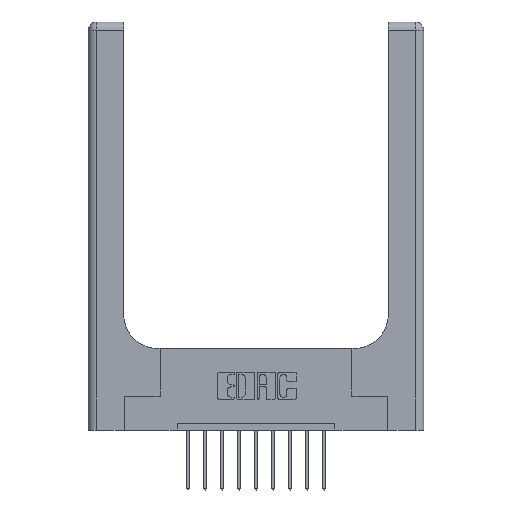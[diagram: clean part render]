
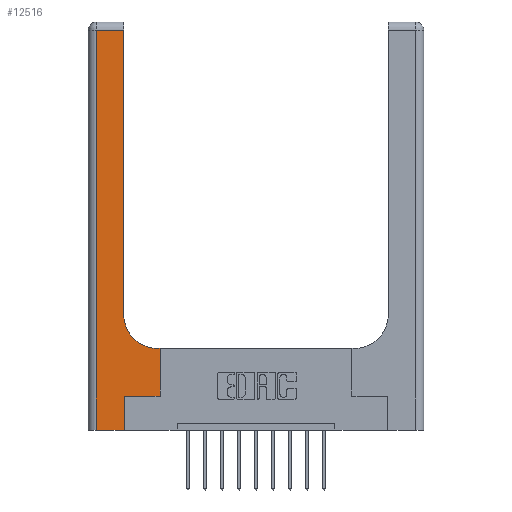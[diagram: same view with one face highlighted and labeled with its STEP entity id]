
A CAD part, top view. The second image highlights one B-rep face of the part: STEP entity #12516.
In plain terms, the highlighted planar face has unit normal (0, 0, 1).
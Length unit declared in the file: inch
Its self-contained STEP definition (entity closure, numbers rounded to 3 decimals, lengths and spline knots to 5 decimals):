
#198 = LINE ( 'NONE', #5008, #10710 ) ;
#617 = DIRECTION ( 'NONE',  ( 0., 0., -1. ) ) ;
#847 = VERTEX_POINT ( 'NONE', #10079 ) ;
#943 = EDGE_CURVE ( 'NONE', #5812, #9775, #3276, .T. ) ;
#958 = EDGE_LOOP ( 'NONE', ( #9670, #5380, #9196, #5825, #5721, #4698, #2646, #11241, #13419 ) ) ;
#1490 = CARTESIAN_POINT ( 'NONE',  ( 0.26, 2.94, 0.37 ) ) ;
#1755 = VERTEX_POINT ( 'NONE', #4124 ) ;
#2217 = LINE ( 'NONE', #7058, #12520 ) ;
#2228 = CARTESIAN_POINT ( 'NONE',  ( 0.265, 0., 0.37 ) ) ;
#2293 = VERTEX_POINT ( 'NONE', #7023 ) ;
#2319 = VECTOR ( 'NONE', #10686, 39.37008 ) ;
#2527 = EDGE_CURVE ( 'NONE', #1755, #2293, #14695, .T. ) ;
#2646 = ORIENTED_EDGE ( 'NONE', *, *, #2527, .T. ) ;
#3151 = LINE ( 'NONE', #15145, #7946 ) ;
#3276 = LINE ( 'NONE', #9407, #2319 ) ;
#3753 = VERTEX_POINT ( 'NONE', #9052 ) ;
#3847 = FACE_OUTER_BOUND ( 'NONE', #958, .T. ) ;
#4062 = VERTEX_POINT ( 'NONE', #7925 ) ;
#4124 = CARTESIAN_POINT ( 'NONE',  ( 0.528, 0.25, 0.37 ) ) ;
#4272 = DIRECTION ( 'NONE',  ( -1., 0., 0. ) ) ;
#4309 = DIRECTION ( 'NONE',  ( -1., 0., 0. ) ) ;
#4390 = CARTESIAN_POINT ( 'NONE',  ( 0.26, 0.6, 0.37 ) ) ;
#4558 = VERTEX_POINT ( 'NONE', #15347 ) ;
#4698 = ORIENTED_EDGE ( 'NONE', *, *, #9239, .T. ) ;
#5008 = CARTESIAN_POINT ( 'NONE',  ( 0., 0., 0.37 ) ) ;
#5085 = DIRECTION ( 'NONE',  ( 0., 1., 0. ) ) ;
#5380 = ORIENTED_EDGE ( 'NONE', *, *, #9116, .T. ) ;
#5564 = LINE ( 'NONE', #2228, #12491 ) ;
#5721 = ORIENTED_EDGE ( 'NONE', *, *, #13725, .T. ) ;
#5812 = VERTEX_POINT ( 'NONE', #6152 ) ;
#5825 = ORIENTED_EDGE ( 'NONE', *, *, #8790, .T. ) ;
#5881 = DIRECTION ( 'NONE',  ( 0., 1., 0. ) ) ;
#6116 = EDGE_CURVE ( 'NONE', #847, #4062, #7657, .T. ) ;
#6152 = CARTESIAN_POINT ( 'NONE',  ( 0.26, 0.85, 0.37 ) ) ;
#6202 = CARTESIAN_POINT ( 'NONE',  ( 0.528, 0.25, 0.37 ) ) ;
#6392 = DIRECTION ( 'NONE',  ( 1., 0., 0. ) ) ;
#6545 = AXIS2_PLACEMENT_3D ( 'NONE', #9834, #13670, #8715 ) ;
#7001 = AXIS2_PLACEMENT_3D ( 'NONE', #10214, #617, #6392 ) ;
#7023 = CARTESIAN_POINT ( 'NONE',  ( 0.528, 0.6, 0.37 ) ) ;
#7058 = CARTESIAN_POINT ( 'NONE',  ( 0.265, 0.25, 0.37 ) ) ;
#7136 = DIRECTION ( 'NONE',  ( 1., 0., 0. ) ) ;
#7339 = LINE ( 'NONE', #4390, #8923 ) ;
#7657 = LINE ( 'NONE', #15008, #14928 ) ;
#7925 = CARTESIAN_POINT ( 'NONE',  ( 0.06, 0., 0.37 ) ) ;
#7946 = VECTOR ( 'NONE', #4272, 39.37008 ) ;
#8444 = VECTOR ( 'NONE', #5085, 39.37008 ) ;
#8715 = DIRECTION ( 'NONE',  ( -1., 0., 0. ) ) ;
#8790 = EDGE_CURVE ( 'NONE', #4062, #3753, #198, .T. ) ;
#8923 = VECTOR ( 'NONE', #4309, 39.37008 ) ;
#9052 = CARTESIAN_POINT ( 'NONE',  ( 0.265, 0., 0.37 ) ) ;
#9116 = EDGE_CURVE ( 'NONE', #9775, #847, #3151, .T. ) ;
#9196 = ORIENTED_EDGE ( 'NONE', *, *, #6116, .T. ) ;
#9239 = EDGE_CURVE ( 'NONE', #12448, #1755, #2217, .T. ) ;
#9407 = CARTESIAN_POINT ( 'NONE',  ( 0.26, 3., 0.37 ) ) ;
#9670 = ORIENTED_EDGE ( 'NONE', *, *, #943, .T. ) ;
#9775 = VERTEX_POINT ( 'NONE', #1490 ) ;
#9834 = CARTESIAN_POINT ( 'NONE',  ( 0., 3., 0.37 ) ) ;
#10079 = CARTESIAN_POINT ( 'NONE',  ( 0.06, 2.94, 0.37 ) ) ;
#10118 = DIRECTION ( 'NONE',  ( 0., -1., 0. ) ) ;
#10214 = CARTESIAN_POINT ( 'NONE',  ( 0.51, 0.85, 0.37 ) ) ;
#10327 = EDGE_CURVE ( 'NONE', #2293, #4558, #7339, .T. ) ;
#10686 = DIRECTION ( 'NONE',  ( 0., 1., 0. ) ) ;
#10710 = VECTOR ( 'NONE', #11302, 39.37008 ) ;
#11241 = ORIENTED_EDGE ( 'NONE', *, *, #10327, .T. ) ;
#11302 = DIRECTION ( 'NONE',  ( 1., 0., 0. ) ) ;
#12383 = CARTESIAN_POINT ( 'NONE',  ( 0.265, 0.25, 0.37 ) ) ;
#12448 = VERTEX_POINT ( 'NONE', #12383 ) ;
#12491 = VECTOR ( 'NONE', #5881, 39.37008 ) ;
#12516 = ADVANCED_FACE ( 'NONE', ( #3847 ), #14817, .F. ) ;
#12520 = VECTOR ( 'NONE', #7136, 39.37008 ) ;
#13103 = EDGE_CURVE ( 'NONE', #4558, #5812, #14611, .T. ) ;
#13419 = ORIENTED_EDGE ( 'NONE', *, *, #13103, .T. ) ;
#13670 = DIRECTION ( 'NONE',  ( 0., 0., -1. ) ) ;
#13725 = EDGE_CURVE ( 'NONE', #3753, #12448, #5564, .T. ) ;
#14611 = CIRCLE ( 'NONE', #7001, 0.25 ) ;
#14695 = LINE ( 'NONE', #6202, #8444 ) ;
#14817 = PLANE ( 'NONE',  #6545 ) ;
#14928 = VECTOR ( 'NONE', #10118, 39.37008 ) ;
#15008 = CARTESIAN_POINT ( 'NONE',  ( 0.06, 3., 0.37 ) ) ;
#15145 = CARTESIAN_POINT ( 'NONE',  ( 0., 2.94, 0.37 ) ) ;
#15347 = CARTESIAN_POINT ( 'NONE',  ( 0.51, 0.6, 0.37 ) ) ;
